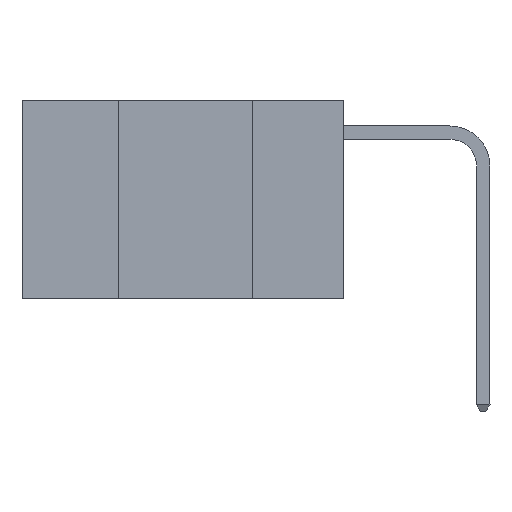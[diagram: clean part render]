
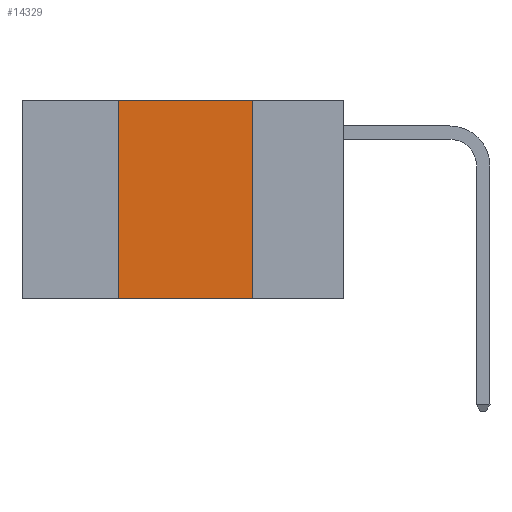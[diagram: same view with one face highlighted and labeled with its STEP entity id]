
A CAD part, left-side view. The second image highlights one B-rep face of the part: STEP entity #14329.
In plain terms, the highlighted planar face has unit normal (-1, 0, 0).
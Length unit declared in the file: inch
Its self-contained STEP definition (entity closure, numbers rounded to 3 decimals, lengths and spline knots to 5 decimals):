
#719 = VECTOR ( 'NONE', #14661, 39.37008 ) ;
#1938 = CARTESIAN_POINT ( 'NONE',  ( 0., 0.17, 0. ) ) ;
#3172 = CARTESIAN_POINT ( 'NONE',  ( 0., 0.42, 0. ) ) ;
#4214 = CARTESIAN_POINT ( 'NONE',  ( 0., 0.6, -0.37 ) ) ;
#4733 = EDGE_CURVE ( 'NONE', #10655, #17143, #12077, .T. ) ;
#6400 = CARTESIAN_POINT ( 'NONE',  ( 0., 0.42, 0. ) ) ;
#6605 = FACE_OUTER_BOUND ( 'NONE', #14490, .T. ) ;
#6647 = CARTESIAN_POINT ( 'NONE',  ( 0., 0.17, -0.37 ) ) ;
#8367 = DIRECTION ( 'NONE',  ( 1., 0., 0. ) ) ;
#9302 = ORIENTED_EDGE ( 'NONE', *, *, #13599, .F. ) ;
#9497 = ORIENTED_EDGE ( 'NONE', *, *, #22152, .F. ) ;
#10655 = VERTEX_POINT ( 'NONE', #18514 ) ;
#10681 = PLANE ( 'NONE',  #11115 ) ;
#11108 = VERTEX_POINT ( 'NONE', #13192 ) ;
#11115 = AXIS2_PLACEMENT_3D ( 'NONE', #19075, #8367, #25035 ) ;
#11823 = LINE ( 'NONE', #22248, #21972 ) ;
#12077 = LINE ( 'NONE', #4214, #22511 ) ;
#12612 = DIRECTION ( 'NONE',  ( 0., 0., -1. ) ) ;
#13192 = CARTESIAN_POINT ( 'NONE',  ( 0., 0.17, 0. ) ) ;
#13599 = EDGE_CURVE ( 'NONE', #10655, #23354, #24965, .T. ) ;
#14329 = ADVANCED_FACE ( 'NONE', ( #6605 ), #10681, .F. ) ;
#14490 = EDGE_LOOP ( 'NONE', ( #9497, #17504, #9302, #21857 ) ) ;
#14661 = DIRECTION ( 'NONE',  ( 0., 0., 1. ) ) ;
#17143 = VERTEX_POINT ( 'NONE', #6647 ) ;
#17504 = ORIENTED_EDGE ( 'NONE', *, *, #25566, .F. ) ;
#18440 = LINE ( 'NONE', #1938, #23643 ) ;
#18514 = CARTESIAN_POINT ( 'NONE',  ( 0., 0.42, -0.37 ) ) ;
#19075 = CARTESIAN_POINT ( 'NONE',  ( 0., 0.6, 0. ) ) ;
#20995 = DIRECTION ( 'NONE',  ( 0., -1., 0. ) ) ;
#21857 = ORIENTED_EDGE ( 'NONE', *, *, #4733, .T. ) ;
#21972 = VECTOR ( 'NONE', #26436, 39.37008 ) ;
#22152 = EDGE_CURVE ( 'NONE', #11108, #17143, #18440, .T. ) ;
#22248 = CARTESIAN_POINT ( 'NONE',  ( 0., 0.6, 0. ) ) ;
#22511 = VECTOR ( 'NONE', #20995, 39.37008 ) ;
#23354 = VERTEX_POINT ( 'NONE', #3172 ) ;
#23643 = VECTOR ( 'NONE', #12612, 39.37008 ) ;
#24965 = LINE ( 'NONE', #6400, #719 ) ;
#25035 = DIRECTION ( 'NONE',  ( 0., 0., -1. ) ) ;
#25566 = EDGE_CURVE ( 'NONE', #23354, #11108, #11823, .T. ) ;
#26436 = DIRECTION ( 'NONE',  ( 0., -1., 0. ) ) ;
